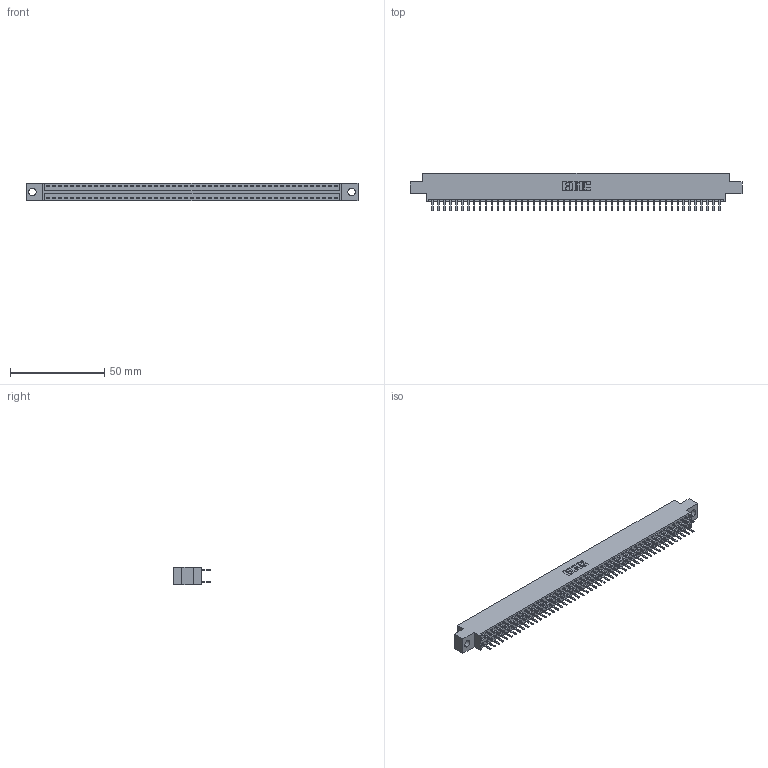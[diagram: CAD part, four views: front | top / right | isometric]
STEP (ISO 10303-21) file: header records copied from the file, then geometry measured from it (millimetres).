
FILE_DESCRIPTION (( 'STEP AP203' ), '1' );
FILE_NAME ('396-098-520-804.STEP', '2019-11-02T16:55:43', ( '' ), ( '' ), 'SwSTEP 2.0', 'SolidWorks 2016', '' );
FILE_SCHEMA (( 'CONFIG_CONTROL_DESIGN' ));
Length unit declared in the file: inch
Products named in the file (3): 346 Part_0.170 Offset - 0.156 Dia-TH; 345-292-001_345-293-120; 396-098-520-804
Assembly tree (99 placements, depth 2):
  396-098-520-804
    346 Part_0.170 Offset - 0.156 Dia-TH
    345-292-001_345-293-120  x98
Bounding box: 176.15 x 20.02 x 9.4 mm (x, y, z)
Volume: 16945.5 mm3; surface area: 23294.8 mm2
Topology: 99 solids, 99 shells, 5614 faces, 16315 edges, 10614 vertices
Faces by surface type: plane 3706, cylinder 1908
Entity records: 31285 total; most frequent: CARTESIAN_POINT 5160, ORIENTED_EDGE 5082, DIRECTION 4585, EDGE_CURVE 2541, VECTOR 2209, LINE 2209, VERTEX_POINT 1690, AXIS2_PLACEMENT_3D 1188
